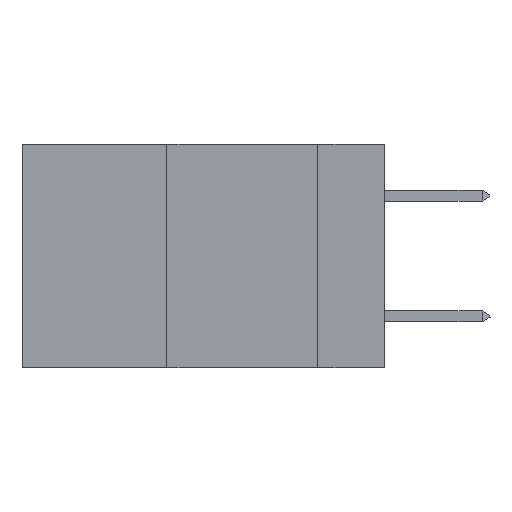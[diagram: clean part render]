
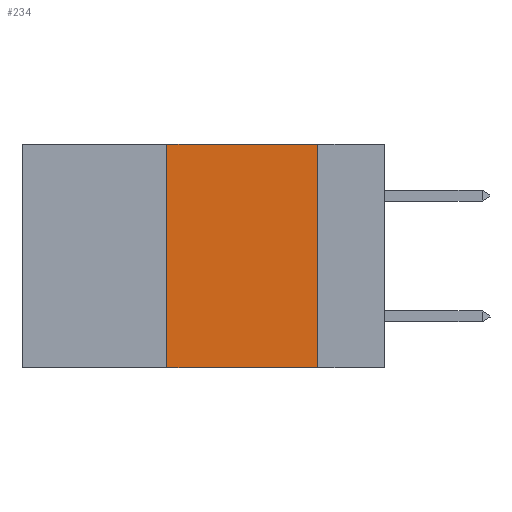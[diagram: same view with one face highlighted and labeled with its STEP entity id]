
A CAD part, left-side view. The second image highlights one B-rep face of the part: STEP entity #234.
In plain terms, the highlighted planar face has unit normal (-1, 0, 0).
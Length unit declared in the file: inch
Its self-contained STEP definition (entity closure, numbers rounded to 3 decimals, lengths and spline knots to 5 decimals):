
#234 = ADVANCED_FACE ( 'NONE', ( #23187 ), #12716, .F. ) ;
#1503 = CARTESIAN_POINT ( 'NONE',  ( 0., 0.11, 0. ) ) ;
#1956 = VERTEX_POINT ( 'NONE', #2518 ) ;
#2120 = ORIENTED_EDGE ( 'NONE', *, *, #20237, .F. ) ;
#2518 = CARTESIAN_POINT ( 'NONE',  ( 0., 0.36, -0.37 ) ) ;
#3099 = DIRECTION ( 'NONE',  ( 1., 0., 0. ) ) ;
#3723 = ORIENTED_EDGE ( 'NONE', *, *, #12694, .F. ) ;
#5056 = VERTEX_POINT ( 'NONE', #22111 ) ;
#5562 = VECTOR ( 'NONE', #6277, 39.37008 ) ;
#5944 = ORIENTED_EDGE ( 'NONE', *, *, #12466, .T. ) ;
#6277 = DIRECTION ( 'NONE',  ( 0., -1., 0. ) ) ;
#6807 = ORIENTED_EDGE ( 'NONE', *, *, #12909, .F. ) ;
#7317 = VERTEX_POINT ( 'NONE', #12165 ) ;
#7344 = LINE ( 'NONE', #7581, #11132 ) ;
#7543 = VERTEX_POINT ( 'NONE', #19125 ) ;
#7581 = CARTESIAN_POINT ( 'NONE',  ( 0., 0.36, 0. ) ) ;
#8744 = DIRECTION ( 'NONE',  ( 0., 0., -1. ) ) ;
#10204 = LINE ( 'NONE', #1503, #14601 ) ;
#10865 = CARTESIAN_POINT ( 'NONE',  ( 0., 0.6, 0. ) ) ;
#11095 = DIRECTION ( 'NONE',  ( 0., 0., 1. ) ) ;
#11132 = VECTOR ( 'NONE', #11095, 39.37008 ) ;
#12165 = CARTESIAN_POINT ( 'NONE',  ( 0., 0.11, 0. ) ) ;
#12466 = EDGE_CURVE ( 'NONE', #1956, #5056, #21497, .T. ) ;
#12694 = EDGE_CURVE ( 'NONE', #1956, #7543, #7344, .T. ) ;
#12716 = PLANE ( 'NONE',  #20956 ) ;
#12909 = EDGE_CURVE ( 'NONE', #7317, #5056, #10204, .T. ) ;
#13744 = EDGE_LOOP ( 'NONE', ( #6807, #2120, #3723, #5944 ) ) ;
#14601 = VECTOR ( 'NONE', #16509, 39.37008 ) ;
#16509 = DIRECTION ( 'NONE',  ( 0., 0., -1. ) ) ;
#16678 = VECTOR ( 'NONE', #21772, 39.37008 ) ;
#16711 = LINE ( 'NONE', #17897, #16678 ) ;
#17897 = CARTESIAN_POINT ( 'NONE',  ( 0., 0.6, 0. ) ) ;
#19125 = CARTESIAN_POINT ( 'NONE',  ( 0., 0.36, 0. ) ) ;
#19152 = CARTESIAN_POINT ( 'NONE',  ( 0., 0.6, -0.37 ) ) ;
#20237 = EDGE_CURVE ( 'NONE', #7543, #7317, #16711, .T. ) ;
#20956 = AXIS2_PLACEMENT_3D ( 'NONE', #10865, #3099, #8744 ) ;
#21497 = LINE ( 'NONE', #19152, #5562 ) ;
#21772 = DIRECTION ( 'NONE',  ( 0., -1., 0. ) ) ;
#22111 = CARTESIAN_POINT ( 'NONE',  ( 0., 0.11, -0.37 ) ) ;
#23187 = FACE_OUTER_BOUND ( 'NONE', #13744, .T. ) ;
